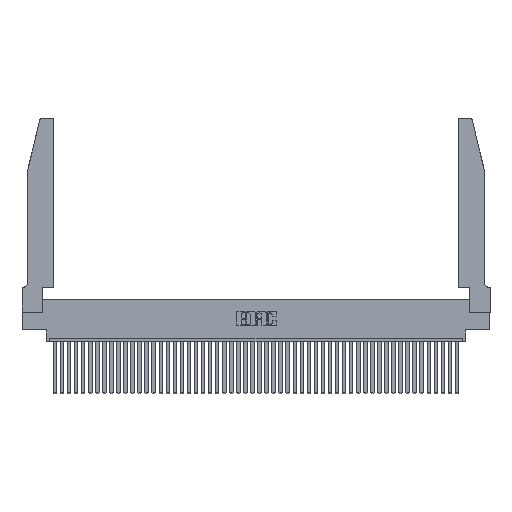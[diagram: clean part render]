
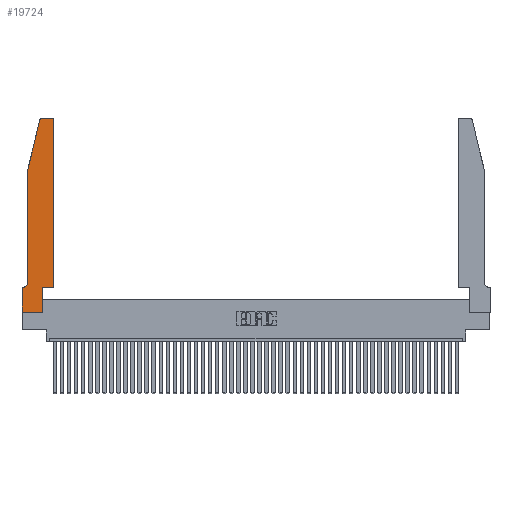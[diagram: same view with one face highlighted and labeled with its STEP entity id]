
A CAD part, top view. The second image highlights one B-rep face of the part: STEP entity #19724.
In plain terms, the highlighted planar face has unit normal (0, 0, 1).
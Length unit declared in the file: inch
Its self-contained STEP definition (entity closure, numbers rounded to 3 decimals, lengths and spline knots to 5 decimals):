
#251 = ORIENTED_EDGE ( 'NONE', *, *, #1863, .T. ) ;
#687 = ORIENTED_EDGE ( 'NONE', *, *, #3282, .T. ) ;
#878 = VECTOR ( 'NONE', #42832, 39.37008 ) ;
#1066 = VECTOR ( 'NONE', #36678, 39.37008 ) ;
#1248 = AXIS2_PLACEMENT_3D ( 'NONE', #32594, #29323, #7889 ) ;
#1604 = CARTESIAN_POINT ( 'NONE',  ( 0.0755, 0.42, 0.37 ) ) ;
#1838 = ORIENTED_EDGE ( 'NONE', *, *, #19155, .T. ) ;
#1863 = EDGE_CURVE ( 'NONE', #8786, #37968, #25604, .T. ) ;
#2157 = EDGE_CURVE ( 'NONE', #10969, #45552, #38998, .T. ) ;
#3212 = DIRECTION ( 'NONE',  ( 0., 0., -1. ) ) ;
#3282 = EDGE_CURVE ( 'NONE', #39898, #5043, #24442, .T. ) ;
#3549 = DIRECTION ( 'NONE',  ( 1., 0., 0. ) ) ;
#3724 = ORIENTED_EDGE ( 'NONE', *, *, #37072, .T. ) ;
#3790 = VECTOR ( 'NONE', #17574, 39.37008 ) ;
#4648 = EDGE_CURVE ( 'NONE', #31092, #8786, #45496, .T. ) ;
#5019 = CARTESIAN_POINT ( 'NONE',  ( 0.4505, 2.72, 0.37 ) ) ;
#5043 = VERTEX_POINT ( 'NONE', #37585 ) ;
#6838 = ORIENTED_EDGE ( 'NONE', *, *, #35265, .T. ) ;
#7058 = CARTESIAN_POINT ( 'NONE',  ( 0.284, 2.75, 0.37 ) ) ;
#7889 = DIRECTION ( 'NONE',  ( 1., 0., 0. ) ) ;
#8786 = VERTEX_POINT ( 'NONE', #1604 ) ;
#9435 = CARTESIAN_POINT ( 'NONE',  ( 0., 0., 0.37 ) ) ;
#9787 = DIRECTION ( 'NONE',  ( 0., 0., 1. ) ) ;
#10137 = CIRCLE ( 'NONE', #25712, 0.03 ) ;
#10367 = CARTESIAN_POINT ( 'NONE',  ( 0.4505, 0.35, 0.37 ) ) ;
#10802 = CARTESIAN_POINT ( 'NONE',  ( 0.0755, 2., 0.37 ) ) ;
#10969 = VERTEX_POINT ( 'NONE', #10367 ) ;
#11309 = CIRCLE ( 'NONE', #11870, 0.03 ) ;
#11870 = AXIS2_PLACEMENT_3D ( 'NONE', #14098, #13951, #3549 ) ;
#11995 = VERTEX_POINT ( 'NONE', #35362 ) ;
#12498 = CARTESIAN_POINT ( 'NONE',  ( 0.2605, 2.75, 0.37 ) ) ;
#12584 = EDGE_LOOP ( 'NONE', ( #42973, #23472, #6838, #20017, #251, #31909, #19408, #687, #33743, #1838, #28909, #3724 ) ) ;
#13200 = CARTESIAN_POINT ( 'NONE',  ( 0.0755, 0.35, 0.37 ) ) ;
#13344 = DIRECTION ( 'NONE',  ( 1., 0., 0. ) ) ;
#13565 = FACE_OUTER_BOUND ( 'NONE', #12584, .T. ) ;
#13576 = DIRECTION ( 'NONE',  ( 1., 0., 0. ) ) ;
#13939 = CARTESIAN_POINT ( 'NONE',  ( 0.4505, 0.35, 0.37 ) ) ;
#13944 = LINE ( 'NONE', #18838, #1066 ) ;
#13951 = DIRECTION ( 'NONE',  ( 0., 0., 1. ) ) ;
#14098 = CARTESIAN_POINT ( 'NONE',  ( 0.4205, 2.72, 0.37 ) ) ;
#14137 = VERTEX_POINT ( 'NONE', #24643 ) ;
#14711 = EDGE_CURVE ( 'NONE', #37871, #31535, #10137, .T. ) ;
#14773 = VECTOR ( 'NONE', #13576, 39.37008 ) ;
#15365 = CARTESIAN_POINT ( 'NONE',  ( 0., 0.35, 0.37 ) ) ;
#15596 = LINE ( 'NONE', #9435, #16783 ) ;
#16104 = LINE ( 'NONE', #12498, #37346 ) ;
#16783 = VECTOR ( 'NONE', #17085, 39.37008 ) ;
#16904 = EDGE_CURVE ( 'NONE', #14137, #37871, #16104, .T. ) ;
#17085 = DIRECTION ( 'NONE',  ( 0., -1., 0. ) ) ;
#17574 = DIRECTION ( 'NONE',  ( 0., 1., 0. ) ) ;
#18681 = CARTESIAN_POINT ( 'NONE',  ( 0.4505, 0.35, 0.37 ) ) ;
#18793 = LINE ( 'NONE', #13200, #30606 ) ;
#18838 = CARTESIAN_POINT ( 'NONE',  ( 0.2865, 0.35, 0.37 ) ) ;
#19155 = EDGE_CURVE ( 'NONE', #11995, #10969, #36565, .T. ) ;
#19408 = ORIENTED_EDGE ( 'NONE', *, *, #23002, .T. ) ;
#19724 = ADVANCED_FACE ( 'NONE', ( #13565 ), #36667, .T. ) ;
#20017 = ORIENTED_EDGE ( 'NONE', *, *, #4648, .T. ) ;
#20140 = DIRECTION ( 'NONE',  ( -1., 0., 0. ) ) ;
#21125 = AXIS2_PLACEMENT_3D ( 'NONE', #31767, #3212, #35370 ) ;
#22125 = DIRECTION ( 'NONE',  ( 1., 0., 0. ) ) ;
#23002 = EDGE_CURVE ( 'NONE', #38009, #39898, #15596, .T. ) ;
#23472 = ORIENTED_EDGE ( 'NONE', *, *, #14711, .T. ) ;
#24442 = LINE ( 'NONE', #42336, #14773 ) ;
#24643 = CARTESIAN_POINT ( 'NONE',  ( 0.4205, 2.75, 0.37 ) ) ;
#25604 = CIRCLE ( 'NONE', #21125, 0.07 ) ;
#25712 = AXIS2_PLACEMENT_3D ( 'NONE', #35123, #9787, #13344 ) ;
#28909 = ORIENTED_EDGE ( 'NONE', *, *, #2157, .T. ) ;
#29323 = DIRECTION ( 'NONE',  ( 0., 0., 1. ) ) ;
#30606 = VECTOR ( 'NONE', #20140, 39.37008 ) ;
#31092 = VERTEX_POINT ( 'NONE', #36777 ) ;
#31535 = VERTEX_POINT ( 'NONE', #36287 ) ;
#31767 = CARTESIAN_POINT ( 'NONE',  ( 0.0055, 0.42, 0.37 ) ) ;
#31909 = ORIENTED_EDGE ( 'NONE', *, *, #39153, .T. ) ;
#32594 = CARTESIAN_POINT ( 'NONE',  ( 0., 0.35, 0.37 ) ) ;
#33674 = DIRECTION ( 'NONE',  ( 0., -1., 0. ) ) ;
#33743 = ORIENTED_EDGE ( 'NONE', *, *, #38977, .T. ) ;
#34932 = VECTOR ( 'NONE', #33674, 39.37008 ) ;
#35123 = CARTESIAN_POINT ( 'NONE',  ( 0.284, 2.72, 0.37 ) ) ;
#35265 = EDGE_CURVE ( 'NONE', #31535, #31092, #38961, .T. ) ;
#35362 = CARTESIAN_POINT ( 'NONE',  ( 0.2865, 0.35, 0.37 ) ) ;
#35370 = DIRECTION ( 'NONE',  ( -1., 0., 0. ) ) ;
#36022 = CARTESIAN_POINT ( 'NONE',  ( 0.0755, 2., 0.37 ) ) ;
#36287 = CARTESIAN_POINT ( 'NONE',  ( 0.25487, 2.72718, 0.37 ) ) ;
#36565 = LINE ( 'NONE', #18681, #44959 ) ;
#36667 = PLANE ( 'NONE',  #1248 ) ;
#36678 = DIRECTION ( 'NONE',  ( 0., 1., 0. ) ) ;
#36777 = CARTESIAN_POINT ( 'NONE',  ( 0.0755, 2., 0.37 ) ) ;
#36843 = CARTESIAN_POINT ( 'NONE',  ( 0.0055, 0.35, 0.37 ) ) ;
#37072 = EDGE_CURVE ( 'NONE', #45552, #14137, #11309, .T. ) ;
#37346 = VECTOR ( 'NONE', #37692, 39.37008 ) ;
#37585 = CARTESIAN_POINT ( 'NONE',  ( 0.2865, 0., 0.37 ) ) ;
#37692 = DIRECTION ( 'NONE',  ( -1., 0., 0. ) ) ;
#37871 = VERTEX_POINT ( 'NONE', #7058 ) ;
#37968 = VERTEX_POINT ( 'NONE', #36843 ) ;
#38009 = VERTEX_POINT ( 'NONE', #15365 ) ;
#38961 = LINE ( 'NONE', #10802, #878 ) ;
#38977 = EDGE_CURVE ( 'NONE', #5043, #11995, #13944, .T. ) ;
#38998 = LINE ( 'NONE', #13939, #3790 ) ;
#39153 = EDGE_CURVE ( 'NONE', #37968, #38009, #18793, .T. ) ;
#39400 = CARTESIAN_POINT ( 'NONE',  ( 0., 0., 0.37 ) ) ;
#39898 = VERTEX_POINT ( 'NONE', #39400 ) ;
#42336 = CARTESIAN_POINT ( 'NONE',  ( 0., 0., 0.37 ) ) ;
#42832 = DIRECTION ( 'NONE',  ( -0.239, -0.971, 0. ) ) ;
#42973 = ORIENTED_EDGE ( 'NONE', *, *, #16904, .T. ) ;
#44959 = VECTOR ( 'NONE', #22125, 39.37008 ) ;
#45496 = LINE ( 'NONE', #36022, #34932 ) ;
#45552 = VERTEX_POINT ( 'NONE', #5019 ) ;
